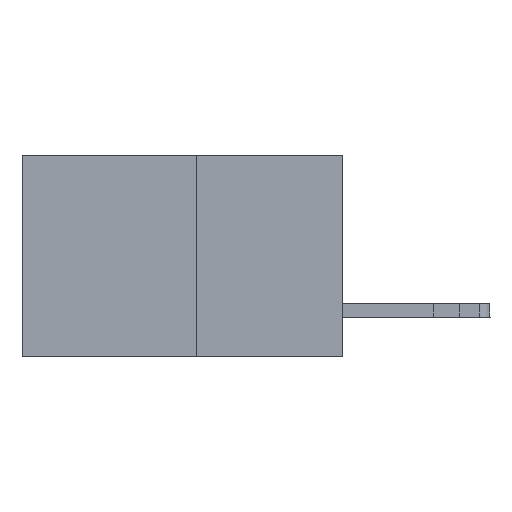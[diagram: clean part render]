
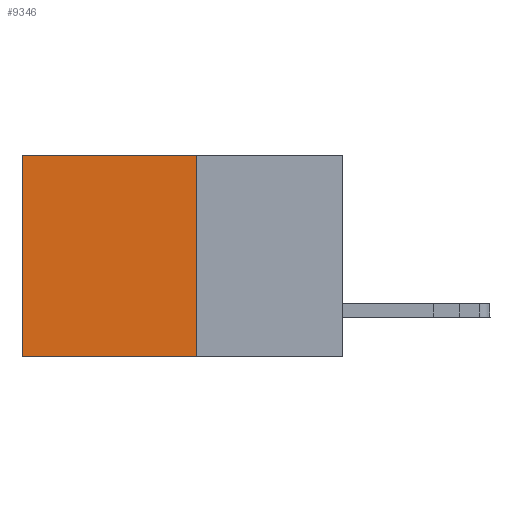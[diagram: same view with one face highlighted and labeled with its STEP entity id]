
A CAD part, left-side view. The second image highlights one B-rep face of the part: STEP entity #9346.
In plain terms, the highlighted planar face has unit normal (-1, 0, 0).
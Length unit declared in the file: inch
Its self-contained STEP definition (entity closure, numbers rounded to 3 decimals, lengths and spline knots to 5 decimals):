
#1327 = DIRECTION ( 'NONE',  ( 0., 0., -1. ) ) ;
#1347 = CARTESIAN_POINT ( 'NONE',  ( 0.277, 0.59, -0.37 ) ) ;
#2066 = DIRECTION ( 'NONE',  ( 0., 1., 0. ) ) ;
#2338 = ORIENTED_EDGE ( 'NONE', *, *, #16587, .F. ) ;
#2407 = CARTESIAN_POINT ( 'NONE',  ( 0.277, 0.27, 0. ) ) ;
#3528 = VECTOR ( 'NONE', #1327, 39.37008 ) ;
#3976 = CARTESIAN_POINT ( 'NONE',  ( 0.277, 0.27, -0.37 ) ) ;
#4357 = VECTOR ( 'NONE', #2066, 39.37008 ) ;
#4671 = VERTEX_POINT ( 'NONE', #2407 ) ;
#4799 = CARTESIAN_POINT ( 'NONE',  ( 0.277, 0.27, 0. ) ) ;
#4883 = CARTESIAN_POINT ( 'NONE',  ( 0.277, 0.59, 0. ) ) ;
#5205 = EDGE_CURVE ( 'NONE', #16651, #19732, #5756, .T. ) ;
#5756 = LINE ( 'NONE', #11907, #3528 ) ;
#6862 = EDGE_CURVE ( 'NONE', #4671, #12622, #19059, .T. ) ;
#7506 = ORIENTED_EDGE ( 'NONE', *, *, #15324, .T. ) ;
#7650 = ORIENTED_EDGE ( 'NONE', *, *, #6862, .F. ) ;
#8249 = ORIENTED_EDGE ( 'NONE', *, *, #5205, .T. ) ;
#9346 = ADVANCED_FACE ( 'NONE', ( #12463 ), #13776, .F. ) ;
#9552 = LINE ( 'NONE', #4799, #18523 ) ;
#10890 = DIRECTION ( 'NONE',  ( 0., 0., -1. ) ) ;
#11162 = DIRECTION ( 'NONE',  ( 0., 1., 0. ) ) ;
#11357 = DIRECTION ( 'NONE',  ( 1., 0., 0. ) ) ;
#11907 = CARTESIAN_POINT ( 'NONE',  ( 0.277, 0.59, -0.37 ) ) ;
#12312 = AXIS2_PLACEMENT_3D ( 'NONE', #3976, #11357, #19015 ) ;
#12463 = FACE_OUTER_BOUND ( 'NONE', #13974, .T. ) ;
#12622 = VERTEX_POINT ( 'NONE', #16749 ) ;
#12956 = LINE ( 'NONE', #14281, #4357 ) ;
#13776 = PLANE ( 'NONE',  #12312 ) ;
#13974 = EDGE_LOOP ( 'NONE', ( #8249, #2338, #7650, #7506 ) ) ;
#14281 = CARTESIAN_POINT ( 'NONE',  ( 0.277, 0.27, -0.37 ) ) ;
#15324 = EDGE_CURVE ( 'NONE', #4671, #16651, #9552, .T. ) ;
#15556 = CARTESIAN_POINT ( 'NONE',  ( 0.277, 0.27, -0.37 ) ) ;
#16587 = EDGE_CURVE ( 'NONE', #12622, #19732, #12956, .T. ) ;
#16651 = VERTEX_POINT ( 'NONE', #4883 ) ;
#16749 = CARTESIAN_POINT ( 'NONE',  ( 0.277, 0.27, -0.37 ) ) ;
#18523 = VECTOR ( 'NONE', #11162, 39.37008 ) ;
#18690 = VECTOR ( 'NONE', #10890, 39.37008 ) ;
#19015 = DIRECTION ( 'NONE',  ( 0., 0., -1. ) ) ;
#19059 = LINE ( 'NONE', #15556, #18690 ) ;
#19732 = VERTEX_POINT ( 'NONE', #1347 ) ;
